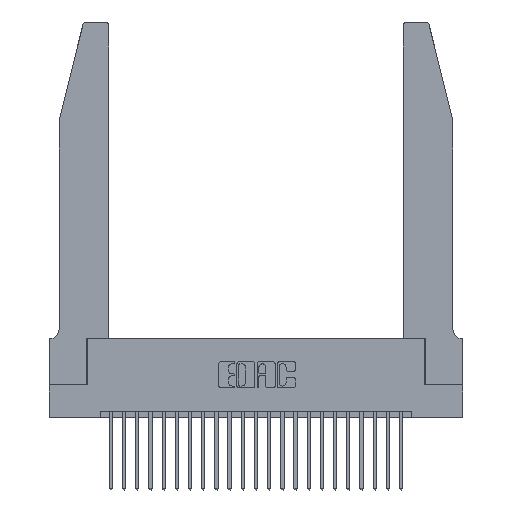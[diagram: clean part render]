
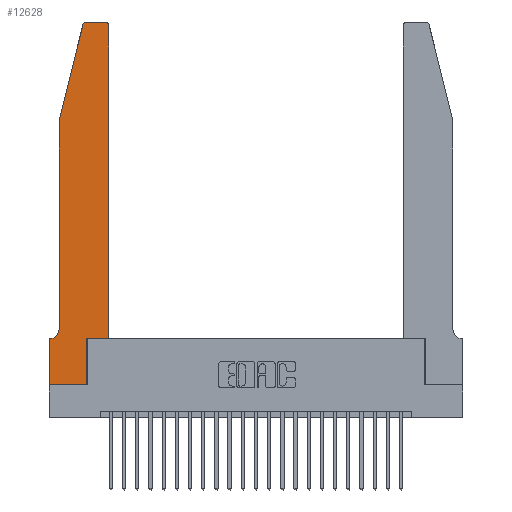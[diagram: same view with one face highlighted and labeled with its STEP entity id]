
A CAD part, top view. The second image highlights one B-rep face of the part: STEP entity #12628.
In plain terms, the highlighted planar face has unit normal (0, 0, 1).
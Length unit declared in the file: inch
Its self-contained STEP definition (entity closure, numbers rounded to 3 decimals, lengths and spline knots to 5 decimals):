
#279 = ORIENTED_EDGE ( 'NONE', *, *, #8222, .T. ) ;
#756 = ORIENTED_EDGE ( 'NONE', *, *, #1837, .T. ) ;
#833 = ORIENTED_EDGE ( 'NONE', *, *, #17563, .T. ) ;
#1099 = CARTESIAN_POINT ( 'NONE',  ( 0.4505, 0.35, 0.37 ) ) ;
#1754 = DIRECTION ( 'NONE',  ( -1., 0., 0. ) ) ;
#1837 = EDGE_CURVE ( 'NONE', #22905, #5038, #13820, .T. ) ;
#1926 = ORIENTED_EDGE ( 'NONE', *, *, #9648, .T. ) ;
#2102 = CARTESIAN_POINT ( 'NONE',  ( 0.0755, 2., 0.37 ) ) ;
#2447 = CARTESIAN_POINT ( 'NONE',  ( 0.284, 2.75, 0.37 ) ) ;
#2549 = DIRECTION ( 'NONE',  ( 0., -1., 0. ) ) ;
#2604 = CARTESIAN_POINT ( 'NONE',  ( 0.0755, 2., 0.37 ) ) ;
#2956 = DIRECTION ( 'NONE',  ( 0., 0., 1. ) ) ;
#3094 = LINE ( 'NONE', #6807, #13137 ) ;
#3150 = VECTOR ( 'NONE', #1754, 39.37008 ) ;
#3168 = DIRECTION ( 'NONE',  ( 0., 0., -1. ) ) ;
#4074 = VECTOR ( 'NONE', #18012, 39.37008 ) ;
#4267 = DIRECTION ( 'NONE',  ( 0., 0., 1. ) ) ;
#4302 = VERTEX_POINT ( 'NONE', #2447 ) ;
#4991 = EDGE_CURVE ( 'NONE', #11962, #17840, #21475, .T. ) ;
#5038 = VERTEX_POINT ( 'NONE', #9300 ) ;
#5070 = ORIENTED_EDGE ( 'NONE', *, *, #16212, .T. ) ;
#5848 = AXIS2_PLACEMENT_3D ( 'NONE', #14245, #4267, #18137 ) ;
#6016 = EDGE_CURVE ( 'NONE', #5038, #6208, #19662, .T. ) ;
#6208 = VERTEX_POINT ( 'NONE', #9234 ) ;
#6333 = VERTEX_POINT ( 'NONE', #9587 ) ;
#6693 = EDGE_CURVE ( 'NONE', #12418, #16983, #24957, .T. ) ;
#6807 = CARTESIAN_POINT ( 'NONE',  ( 0.2605, 2.75, 0.37 ) ) ;
#7332 = DIRECTION ( 'NONE',  ( 0., 0., 1. ) ) ;
#8017 = CARTESIAN_POINT ( 'NONE',  ( 0.4505, 0.35, 0.37 ) ) ;
#8222 = EDGE_CURVE ( 'NONE', #22500, #11962, #18581, .T. ) ;
#8381 = EDGE_CURVE ( 'NONE', #16983, #21770, #9681, .T. ) ;
#8406 = EDGE_CURVE ( 'NONE', #4302, #12418, #19474, .T. ) ;
#8640 = VECTOR ( 'NONE', #2549, 39.37008 ) ;
#8757 = VECTOR ( 'NONE', #24522, 39.37008 ) ;
#8865 = DIRECTION ( 'NONE',  ( -1., 0., 0. ) ) ;
#8891 = CARTESIAN_POINT ( 'NONE',  ( 0.0755, 0.35, 0.37 ) ) ;
#8923 = VECTOR ( 'NONE', #14595, 39.37008 ) ;
#9234 = CARTESIAN_POINT ( 'NONE',  ( 0., 0., 0.37 ) ) ;
#9300 = CARTESIAN_POINT ( 'NONE',  ( 0., 0.35, 0.37 ) ) ;
#9587 = CARTESIAN_POINT ( 'NONE',  ( 0.4205, 2.75, 0.37 ) ) ;
#9648 = EDGE_CURVE ( 'NONE', #21770, #22905, #10546, .T. ) ;
#9681 = LINE ( 'NONE', #23032, #24478 ) ;
#9980 = LINE ( 'NONE', #23851, #25368 ) ;
#10493 = CARTESIAN_POINT ( 'NONE',  ( 0.0055, 0.35, 0.37 ) ) ;
#10546 = CIRCLE ( 'NONE', #22020, 0.07 ) ;
#10981 = ORIENTED_EDGE ( 'NONE', *, *, #4991, .T. ) ;
#11180 = VECTOR ( 'NONE', #13142, 39.37008 ) ;
#11398 = CARTESIAN_POINT ( 'NONE',  ( 0.2865, 0.35, 0.37 ) ) ;
#11962 = VERTEX_POINT ( 'NONE', #8017 ) ;
#12113 = CARTESIAN_POINT ( 'NONE',  ( 0., 0., 0.37 ) ) ;
#12330 = AXIS2_PLACEMENT_3D ( 'NONE', #14936, #2956, #16868 ) ;
#12418 = VERTEX_POINT ( 'NONE', #19402 ) ;
#12628 = ADVANCED_FACE ( 'NONE', ( #21616 ), #16189, .T. ) ;
#13069 = CARTESIAN_POINT ( 'NONE',  ( 0.4505, 0.35, 0.37 ) ) ;
#13137 = VECTOR ( 'NONE', #8865, 39.37008 ) ;
#13142 = DIRECTION ( 'NONE',  ( 0., 1., 0. ) ) ;
#13665 = CARTESIAN_POINT ( 'NONE',  ( 0.0755, 0.42, 0.37 ) ) ;
#13820 = LINE ( 'NONE', #8891, #3150 ) ;
#14242 = ORIENTED_EDGE ( 'NONE', *, *, #24808, .T. ) ;
#14245 = CARTESIAN_POINT ( 'NONE',  ( 0., 0.35, 0.37 ) ) ;
#14359 = ORIENTED_EDGE ( 'NONE', *, *, #8406, .T. ) ;
#14595 = DIRECTION ( 'NONE',  ( -0.239, -0.971, 0. ) ) ;
#14752 = AXIS2_PLACEMENT_3D ( 'NONE', #19105, #7332, #21000 ) ;
#14936 = CARTESIAN_POINT ( 'NONE',  ( 0.284, 2.72, 0.37 ) ) ;
#15133 = CARTESIAN_POINT ( 'NONE',  ( 0.0055, 0.42, 0.37 ) ) ;
#15213 = ORIENTED_EDGE ( 'NONE', *, *, #24035, .T. ) ;
#16189 = PLANE ( 'NONE',  #5848 ) ;
#16212 = EDGE_CURVE ( 'NONE', #17840, #6333, #23661, .T. ) ;
#16474 = CARTESIAN_POINT ( 'NONE',  ( 0., 0., 0.37 ) ) ;
#16776 = DIRECTION ( 'NONE',  ( 0., -1., 0. ) ) ;
#16868 = DIRECTION ( 'NONE',  ( 1., 0., 0. ) ) ;
#16983 = VERTEX_POINT ( 'NONE', #2102 ) ;
#17063 = DIRECTION ( 'NONE',  ( -1., 0., 0. ) ) ;
#17563 = EDGE_CURVE ( 'NONE', #23417, #22500, #9980, .T. ) ;
#17816 = EDGE_LOOP ( 'NONE', ( #14242, #14359, #19160, #19092, #1926, #756, #18814, #15213, #833, #279, #10981, #5070 ) ) ;
#17840 = VERTEX_POINT ( 'NONE', #18984 ) ;
#18012 = DIRECTION ( 'NONE',  ( 1., 0., 0. ) ) ;
#18137 = DIRECTION ( 'NONE',  ( 1., 0., 0. ) ) ;
#18581 = LINE ( 'NONE', #13069, #8757 ) ;
#18814 = ORIENTED_EDGE ( 'NONE', *, *, #6016, .T. ) ;
#18984 = CARTESIAN_POINT ( 'NONE',  ( 0.4505, 2.72, 0.37 ) ) ;
#19092 = ORIENTED_EDGE ( 'NONE', *, *, #8381, .T. ) ;
#19105 = CARTESIAN_POINT ( 'NONE',  ( 0.4205, 2.72, 0.37 ) ) ;
#19160 = ORIENTED_EDGE ( 'NONE', *, *, #6693, .T. ) ;
#19402 = CARTESIAN_POINT ( 'NONE',  ( 0.25487, 2.72718, 0.37 ) ) ;
#19474 = CIRCLE ( 'NONE', #12330, 0.03 ) ;
#19662 = LINE ( 'NONE', #16474, #8640 ) ;
#21000 = DIRECTION ( 'NONE',  ( 1., 0., 0. ) ) ;
#21475 = LINE ( 'NONE', #1099, #11180 ) ;
#21616 = FACE_OUTER_BOUND ( 'NONE', #17816, .T. ) ;
#21770 = VERTEX_POINT ( 'NONE', #13665 ) ;
#22018 = DIRECTION ( 'NONE',  ( 0., 1., 0. ) ) ;
#22020 = AXIS2_PLACEMENT_3D ( 'NONE', #15133, #3168, #17063 ) ;
#22500 = VERTEX_POINT ( 'NONE', #11398 ) ;
#22905 = VERTEX_POINT ( 'NONE', #10493 ) ;
#23032 = CARTESIAN_POINT ( 'NONE',  ( 0.0755, 2., 0.37 ) ) ;
#23417 = VERTEX_POINT ( 'NONE', #23740 ) ;
#23661 = CIRCLE ( 'NONE', #14752, 0.03 ) ;
#23740 = CARTESIAN_POINT ( 'NONE',  ( 0.2865, 0., 0.37 ) ) ;
#23851 = CARTESIAN_POINT ( 'NONE',  ( 0.2865, 0.35, 0.37 ) ) ;
#24035 = EDGE_CURVE ( 'NONE', #6208, #23417, #24855, .T. ) ;
#24478 = VECTOR ( 'NONE', #16776, 39.37008 ) ;
#24522 = DIRECTION ( 'NONE',  ( 1., 0., 0. ) ) ;
#24808 = EDGE_CURVE ( 'NONE', #6333, #4302, #3094, .T. ) ;
#24855 = LINE ( 'NONE', #12113, #4074 ) ;
#24957 = LINE ( 'NONE', #2604, #8923 ) ;
#25368 = VECTOR ( 'NONE', #22018, 39.37008 ) ;
